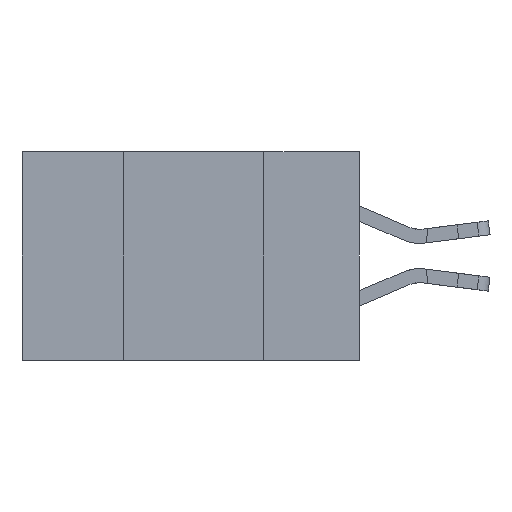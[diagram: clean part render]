
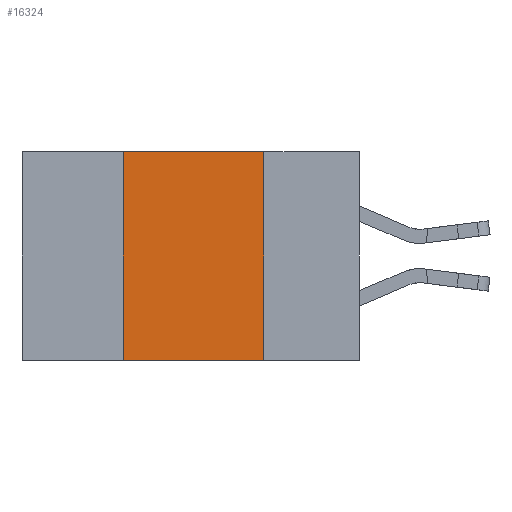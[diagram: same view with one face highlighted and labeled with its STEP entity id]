
A CAD part, left-side view. The second image highlights one B-rep face of the part: STEP entity #16324.
In plain terms, the highlighted planar face has unit normal (-1, 0, 0).
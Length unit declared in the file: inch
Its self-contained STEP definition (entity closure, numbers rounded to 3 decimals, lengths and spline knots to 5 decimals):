
#1340 = PLANE ( 'NONE',  #2274 ) ;
#1747 = ORIENTED_EDGE ( 'NONE', *, *, #17047, .F. ) ;
#2220 = CARTESIAN_POINT ( 'NONE',  ( 0., 0.17, 0. ) ) ;
#2274 = AXIS2_PLACEMENT_3D ( 'NONE', #3709, #24647, #5482 ) ;
#3297 = LINE ( 'NONE', #3534, #8384 ) ;
#3534 = CARTESIAN_POINT ( 'NONE',  ( 0., 0.6, 0. ) ) ;
#3610 = VECTOR ( 'NONE', #17913, 39.37008 ) ;
#3709 = CARTESIAN_POINT ( 'NONE',  ( 0., 0.6, 0. ) ) ;
#5270 = CARTESIAN_POINT ( 'NONE',  ( 0., 0.42, 0. ) ) ;
#5312 = EDGE_CURVE ( 'NONE', #7601, #16505, #6193, .T. ) ;
#5482 = DIRECTION ( 'NONE',  ( 0., 0., -1. ) ) ;
#6193 = LINE ( 'NONE', #8306, #18360 ) ;
#6657 = CARTESIAN_POINT ( 'NONE',  ( 0., 0.6, -0.37 ) ) ;
#6902 = LINE ( 'NONE', #5270, #16718 ) ;
#7601 = VERTEX_POINT ( 'NONE', #2220 ) ;
#8041 = LINE ( 'NONE', #6657, #3610 ) ;
#8067 = ORIENTED_EDGE ( 'NONE', *, *, #23434, .F. ) ;
#8306 = CARTESIAN_POINT ( 'NONE',  ( 0., 0.17, 0. ) ) ;
#8384 = VECTOR ( 'NONE', #11180, 39.37008 ) ;
#8910 = ORIENTED_EDGE ( 'NONE', *, *, #19324, .T. ) ;
#9715 = CARTESIAN_POINT ( 'NONE',  ( 0., 0.17, -0.37 ) ) ;
#11180 = DIRECTION ( 'NONE',  ( 0., -1., 0. ) ) ;
#15697 = CARTESIAN_POINT ( 'NONE',  ( 0., 0.42, 0. ) ) ;
#16324 = ADVANCED_FACE ( 'NONE', ( #16854 ), #1340, .F. ) ;
#16505 = VERTEX_POINT ( 'NONE', #9715 ) ;
#16718 = VECTOR ( 'NONE', #18161, 39.37008 ) ;
#16854 = FACE_OUTER_BOUND ( 'NONE', #19621, .T. ) ;
#17047 = EDGE_CURVE ( 'NONE', #24391, #18142, #6902, .T. ) ;
#17674 = ORIENTED_EDGE ( 'NONE', *, *, #5312, .F. ) ;
#17817 = DIRECTION ( 'NONE',  ( 0., 0., -1. ) ) ;
#17913 = DIRECTION ( 'NONE',  ( 0., -1., 0. ) ) ;
#18142 = VERTEX_POINT ( 'NONE', #15697 ) ;
#18161 = DIRECTION ( 'NONE',  ( 0., 0., 1. ) ) ;
#18360 = VECTOR ( 'NONE', #17817, 39.37008 ) ;
#19324 = EDGE_CURVE ( 'NONE', #24391, #16505, #8041, .T. ) ;
#19621 = EDGE_LOOP ( 'NONE', ( #17674, #8067, #1747, #8910 ) ) ;
#23108 = CARTESIAN_POINT ( 'NONE',  ( 0., 0.42, -0.37 ) ) ;
#23434 = EDGE_CURVE ( 'NONE', #18142, #7601, #3297, .T. ) ;
#24391 = VERTEX_POINT ( 'NONE', #23108 ) ;
#24647 = DIRECTION ( 'NONE',  ( 1., 0., 0. ) ) ;
